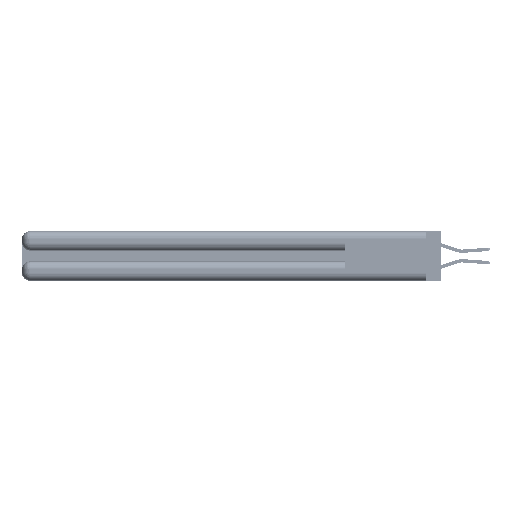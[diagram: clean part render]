
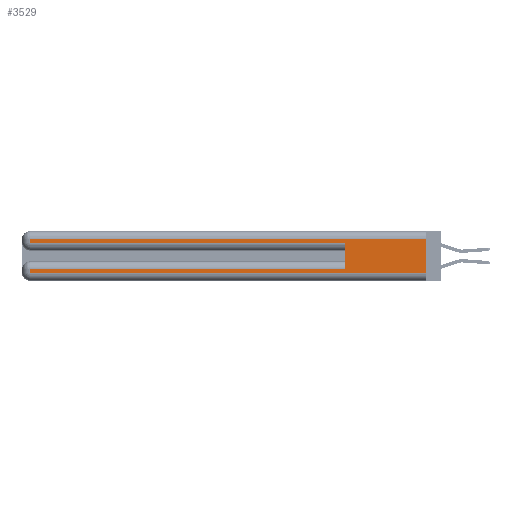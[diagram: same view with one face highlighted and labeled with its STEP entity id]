
A CAD part, left-side view. The second image highlights one B-rep face of the part: STEP entity #3529.
In plain terms, the highlighted planar face has unit normal (-1, 0, 0).
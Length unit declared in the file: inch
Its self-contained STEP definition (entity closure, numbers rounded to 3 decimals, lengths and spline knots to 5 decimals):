
#474 = DIRECTION ( 'NONE',  ( 1., 0., 0. ) ) ;
#1290 = CARTESIAN_POINT ( 'NONE',  ( 0., 0.6, 0.145 ) ) ;
#1389 = EDGE_CURVE ( 'NONE', #8922, #37549, #18745, .T. ) ;
#2100 = CARTESIAN_POINT ( 'NONE',  ( 0., 2.94, 0.285 ) ) ;
#2614 = DIRECTION ( 'NONE',  ( 0., 1., 0. ) ) ;
#3529 = ADVANCED_FACE ( 'NONE', ( #44854 ), #24106, .F. ) ;
#3745 = LINE ( 'NONE', #14517, #29488 ) ;
#3913 = EDGE_CURVE ( 'NONE', #36866, #44399, #31378, .T. ) ;
#4408 = DIRECTION ( 'NONE',  ( 0., 0., -1. ) ) ;
#4691 = VECTOR ( 'NONE', #43431, 39.37008 ) ;
#5938 = CARTESIAN_POINT ( 'NONE',  ( 0., 0., 0.31 ) ) ;
#6255 = LINE ( 'NONE', #19646, #47922 ) ;
#6954 = ORIENTED_EDGE ( 'NONE', *, *, #1389, .T. ) ;
#7359 = CARTESIAN_POINT ( 'NONE',  ( 0., 0., 0.06 ) ) ;
#7429 = VERTEX_POINT ( 'NONE', #5938 ) ;
#8922 = VERTEX_POINT ( 'NONE', #11599 ) ;
#9317 = ORIENTED_EDGE ( 'NONE', *, *, #31836, .T. ) ;
#10061 = ORIENTED_EDGE ( 'NONE', *, *, #17473, .F. ) ;
#10287 = CARTESIAN_POINT ( 'NONE',  ( 0., 0., 0.06 ) ) ;
#10724 = LINE ( 'NONE', #23538, #47508 ) ;
#11599 = CARTESIAN_POINT ( 'NONE',  ( 0., 0.6, 0.085 ) ) ;
#11699 = EDGE_LOOP ( 'NONE', ( #42140, #35930, #9317, #23725, #10061, #6954, #46606, #30723 ) ) ;
#14517 = CARTESIAN_POINT ( 'NONE',  ( 0., 0., 0.31 ) ) ;
#17473 = EDGE_CURVE ( 'NONE', #8922, #49875, #20460, .T. ) ;
#18695 = VECTOR ( 'NONE', #42136, 39.37008 ) ;
#18745 = LINE ( 'NONE', #31994, #4691 ) ;
#19252 = CARTESIAN_POINT ( 'NONE',  ( 0., 2.94, 0.085 ) ) ;
#19646 = CARTESIAN_POINT ( 'NONE',  ( 0., 0., 0.37 ) ) ;
#20401 = DIRECTION ( 'NONE',  ( 0., 0., 1. ) ) ;
#20460 = LINE ( 'NONE', #1290, #24212 ) ;
#21780 = LINE ( 'NONE', #34940, #18695 ) ;
#22467 = EDGE_CURVE ( 'NONE', #7429, #28269, #3745, .T. ) ;
#23257 = VECTOR ( 'NONE', #36366, 39.37008 ) ;
#23538 = CARTESIAN_POINT ( 'NONE',  ( 0., 2.94, 0.37 ) ) ;
#23725 = ORIENTED_EDGE ( 'NONE', *, *, #26889, .T. ) ;
#24106 = PLANE ( 'NONE',  #32148 ) ;
#24212 = VECTOR ( 'NONE', #20401, 39.37008 ) ;
#26889 = EDGE_CURVE ( 'NONE', #33385, #49875, #38568, .T. ) ;
#27072 = VECTOR ( 'NONE', #50189, 39.37008 ) ;
#27719 = DIRECTION ( 'NONE',  ( 0., 0., -1. ) ) ;
#28269 = VERTEX_POINT ( 'NONE', #49726 ) ;
#28773 = EDGE_CURVE ( 'NONE', #37549, #36866, #21780, .T. ) ;
#29488 = VECTOR ( 'NONE', #2614, 39.37008 ) ;
#30639 = EDGE_CURVE ( 'NONE', #7429, #44399, #6255, .T. ) ;
#30723 = ORIENTED_EDGE ( 'NONE', *, *, #3913, .T. ) ;
#31378 = LINE ( 'NONE', #7359, #27072 ) ;
#31836 = EDGE_CURVE ( 'NONE', #28269, #33385, #10724, .T. ) ;
#31994 = CARTESIAN_POINT ( 'NONE',  ( 0., 0., 0.085 ) ) ;
#32148 = AXIS2_PLACEMENT_3D ( 'NONE', #43416, #474, #4408 ) ;
#32696 = CARTESIAN_POINT ( 'NONE',  ( 0., 0.6, 0.285 ) ) ;
#33385 = VERTEX_POINT ( 'NONE', #2100 ) ;
#34940 = CARTESIAN_POINT ( 'NONE',  ( 0., 2.94, 0.37 ) ) ;
#35673 = DIRECTION ( 'NONE',  ( 0., 0., -1. ) ) ;
#35930 = ORIENTED_EDGE ( 'NONE', *, *, #22467, .T. ) ;
#36366 = DIRECTION ( 'NONE',  ( 0., -1., 0. ) ) ;
#36866 = VERTEX_POINT ( 'NONE', #46548 ) ;
#37549 = VERTEX_POINT ( 'NONE', #19252 ) ;
#38568 = LINE ( 'NONE', #48205, #23257 ) ;
#42136 = DIRECTION ( 'NONE',  ( 0., 0., -1. ) ) ;
#42140 = ORIENTED_EDGE ( 'NONE', *, *, #30639, .F. ) ;
#43416 = CARTESIAN_POINT ( 'NONE',  ( 0., 0., 0.37 ) ) ;
#43431 = DIRECTION ( 'NONE',  ( 0., 1., 0. ) ) ;
#44399 = VERTEX_POINT ( 'NONE', #10287 ) ;
#44854 = FACE_OUTER_BOUND ( 'NONE', #11699, .T. ) ;
#46548 = CARTESIAN_POINT ( 'NONE',  ( 0., 2.94, 0.06 ) ) ;
#46606 = ORIENTED_EDGE ( 'NONE', *, *, #28773, .T. ) ;
#47508 = VECTOR ( 'NONE', #35673, 39.37008 ) ;
#47922 = VECTOR ( 'NONE', #27719, 39.37008 ) ;
#48205 = CARTESIAN_POINT ( 'NONE',  ( 0., 0., 0.285 ) ) ;
#49726 = CARTESIAN_POINT ( 'NONE',  ( 0., 2.94, 0.31 ) ) ;
#49875 = VERTEX_POINT ( 'NONE', #32696 ) ;
#50189 = DIRECTION ( 'NONE',  ( 0., -1., 0. ) ) ;
